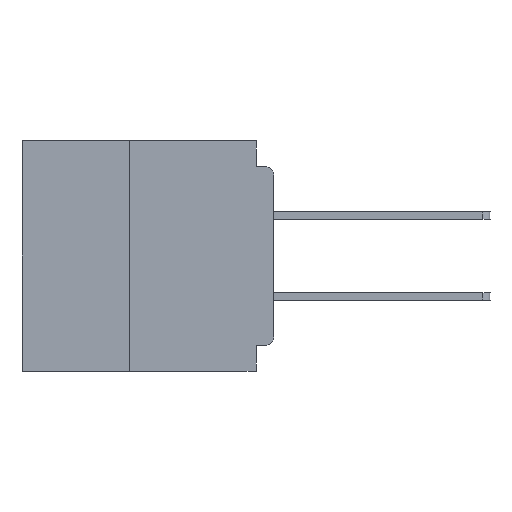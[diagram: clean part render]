
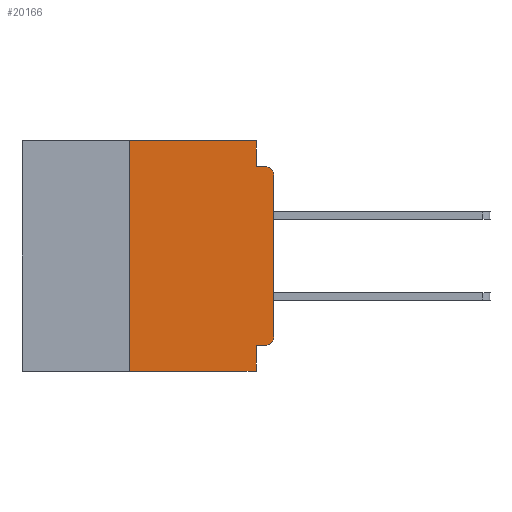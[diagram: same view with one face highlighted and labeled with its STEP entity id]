
A CAD part, left-side view. The second image highlights one B-rep face of the part: STEP entity #20166.
In plain terms, the highlighted planar face has unit normal (-1, 0, 0).
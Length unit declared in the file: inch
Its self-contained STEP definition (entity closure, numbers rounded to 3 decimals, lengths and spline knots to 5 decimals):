
#476 = LINE ( 'NONE', #1852, #50557 ) ;
#1852 = CARTESIAN_POINT ( 'NONE',  ( 0., 0., -0.045 ) ) ;
#2115 = LINE ( 'NONE', #36348, #13239 ) ;
#3683 = ORIENTED_EDGE ( 'NONE', *, *, #18049, .F. ) ;
#3748 = DIRECTION ( 'NONE',  ( 0., 0., -1. ) ) ;
#5530 = EDGE_CURVE ( 'NONE', #58319, #38125, #32464, .T. ) ;
#6383 = ORIENTED_EDGE ( 'NONE', *, *, #33897, .F. ) ;
#6717 = CARTESIAN_POINT ( 'NONE',  ( 0., 0.015, -0.06 ) ) ;
#7727 = VERTEX_POINT ( 'NONE', #37178 ) ;
#9833 = VERTEX_POINT ( 'NONE', #34770 ) ;
#11238 = AXIS2_PLACEMENT_3D ( 'NONE', #6717, #39613, #11486 ) ;
#11486 = DIRECTION ( 'NONE',  ( 0., 0., -1. ) ) ;
#11518 = PLANE ( 'NONE',  #14232 ) ;
#11727 = DIRECTION ( 'NONE',  ( 1., 0., 0. ) ) ;
#12824 = ORIENTED_EDGE ( 'NONE', *, *, #24690, .F. ) ;
#12904 = DIRECTION ( 'NONE',  ( 0., 0., 1. ) ) ;
#13239 = VECTOR ( 'NONE', #12904, 39.37008 ) ;
#14232 = AXIS2_PLACEMENT_3D ( 'NONE', #39861, #11727, #44609 ) ;
#14449 = EDGE_CURVE ( 'NONE', #38474, #18410, #53493, .T. ) ;
#15130 = LINE ( 'NONE', #49622, #51129 ) ;
#15478 = CARTESIAN_POINT ( 'NONE',  ( 0., 0.437, 0. ) ) ;
#16047 = VECTOR ( 'NONE', #32780, 39.37008 ) ;
#17974 = CARTESIAN_POINT ( 'NONE',  ( 0., 0., -0.34 ) ) ;
#18049 = EDGE_CURVE ( 'NONE', #27854, #38474, #33730, .T. ) ;
#18345 = CARTESIAN_POINT ( 'NONE',  ( 0., 0.031, -0.045 ) ) ;
#18410 = VERTEX_POINT ( 'NONE', #18345 ) ;
#18958 = VERTEX_POINT ( 'NONE', #45172 ) ;
#19002 = VECTOR ( 'NONE', #26247, 39.37008 ) ;
#19877 = ORIENTED_EDGE ( 'NONE', *, *, #5530, .T. ) ;
#19957 = VECTOR ( 'NONE', #43953, 39.37008 ) ;
#20166 = ADVANCED_FACE ( 'NONE', ( #29675 ), #11518, .F. ) ;
#21544 = CARTESIAN_POINT ( 'NONE',  ( 0., 0.437, -0.4 ) ) ;
#23103 = AXIS2_PLACEMENT_3D ( 'NONE', #60056, #32019, #3748 ) ;
#23382 = CARTESIAN_POINT ( 'NONE',  ( 0., 0.031, -0.4 ) ) ;
#24259 = EDGE_CURVE ( 'NONE', #9833, #18958, #37246, .T. ) ;
#24690 = EDGE_CURVE ( 'NONE', #54977, #9833, #15130, .T. ) ;
#26247 = DIRECTION ( 'NONE',  ( 0., -1., 0. ) ) ;
#27854 = VERTEX_POINT ( 'NONE', #60236 ) ;
#28115 = DIRECTION ( 'NONE',  ( 0., 0., -1. ) ) ;
#28841 = ORIENTED_EDGE ( 'NONE', *, *, #14449, .F. ) ;
#28901 = ORIENTED_EDGE ( 'NONE', *, *, #60547, .T. ) ;
#29675 = FACE_OUTER_BOUND ( 'NONE', #30309, .T. ) ;
#29832 = CARTESIAN_POINT ( 'NONE',  ( 0., 0., 0. ) ) ;
#30309 = EDGE_LOOP ( 'NONE', ( #19877, #57716, #59818, #28841, #3683, #6383, #57523, #32238, #12824, #28901 ) ) ;
#32019 = DIRECTION ( 'NONE',  ( -1., 0., 0. ) ) ;
#32238 = ORIENTED_EDGE ( 'NONE', *, *, #24259, .F. ) ;
#32464 = LINE ( 'NONE', #29832, #19957 ) ;
#32780 = DIRECTION ( 'NONE',  ( 0., 0., -1. ) ) ;
#33730 = LINE ( 'NONE', #15478, #55713 ) ;
#33897 = EDGE_CURVE ( 'NONE', #45849, #27854, #2115, .T. ) ;
#34366 = EDGE_CURVE ( 'NONE', #38125, #7727, #38171, .T. ) ;
#34408 = DIRECTION ( 'NONE',  ( 0., -1., 0. ) ) ;
#34770 = CARTESIAN_POINT ( 'NONE',  ( 0., 0.031, -0.355 ) ) ;
#34852 = DIRECTION ( 'NONE',  ( 0., -1., 0. ) ) ;
#35163 = CIRCLE ( 'NONE', #23103, 0.015 ) ;
#35776 = VECTOR ( 'NONE', #28115, 39.37008 ) ;
#36348 = CARTESIAN_POINT ( 'NONE',  ( 0., 0.25, -0.4 ) ) ;
#37178 = CARTESIAN_POINT ( 'NONE',  ( 0., 0.015, -0.045 ) ) ;
#37246 = LINE ( 'NONE', #23382, #35776 ) ;
#38125 = VERTEX_POINT ( 'NONE', #47566 ) ;
#38171 = CIRCLE ( 'NONE', #11238, 0.015 ) ;
#38474 = VERTEX_POINT ( 'NONE', #45460 ) ;
#39613 = DIRECTION ( 'NONE',  ( -1., 0., 0. ) ) ;
#39861 = CARTESIAN_POINT ( 'NONE',  ( 0., 0.437, 0. ) ) ;
#40122 = EDGE_CURVE ( 'NONE', #18410, #7727, #476, .T. ) ;
#42158 = CARTESIAN_POINT ( 'NONE',  ( 0., 0.031, 0. ) ) ;
#43953 = DIRECTION ( 'NONE',  ( 0., 0., 1. ) ) ;
#44609 = DIRECTION ( 'NONE',  ( 0., 0., -1. ) ) ;
#45172 = CARTESIAN_POINT ( 'NONE',  ( 0., 0.031, -0.4 ) ) ;
#45318 = CARTESIAN_POINT ( 'NONE',  ( 0., 0.015, -0.355 ) ) ;
#45460 = CARTESIAN_POINT ( 'NONE',  ( 0., 0.031, 0. ) ) ;
#45849 = VERTEX_POINT ( 'NONE', #54045 ) ;
#47566 = CARTESIAN_POINT ( 'NONE',  ( 0., 0., -0.06 ) ) ;
#49622 = CARTESIAN_POINT ( 'NONE',  ( 0., 0., -0.355 ) ) ;
#50557 = VECTOR ( 'NONE', #34852, 39.37008 ) ;
#51129 = VECTOR ( 'NONE', #54321, 39.37008 ) ;
#53493 = LINE ( 'NONE', #42158, #16047 ) ;
#54045 = CARTESIAN_POINT ( 'NONE',  ( 0., 0.25, -0.4 ) ) ;
#54321 = DIRECTION ( 'NONE',  ( 0., 1., 0. ) ) ;
#54977 = VERTEX_POINT ( 'NONE', #45318 ) ;
#55713 = VECTOR ( 'NONE', #34408, 39.37008 ) ;
#56421 = LINE ( 'NONE', #21544, #19002 ) ;
#57523 = ORIENTED_EDGE ( 'NONE', *, *, #60379, .T. ) ;
#57716 = ORIENTED_EDGE ( 'NONE', *, *, #34366, .T. ) ;
#58319 = VERTEX_POINT ( 'NONE', #17974 ) ;
#59818 = ORIENTED_EDGE ( 'NONE', *, *, #40122, .F. ) ;
#60056 = CARTESIAN_POINT ( 'NONE',  ( 0., 0.015, -0.34 ) ) ;
#60236 = CARTESIAN_POINT ( 'NONE',  ( 0., 0.25, 0. ) ) ;
#60379 = EDGE_CURVE ( 'NONE', #45849, #18958, #56421, .T. ) ;
#60547 = EDGE_CURVE ( 'NONE', #54977, #58319, #35163, .T. ) ;
